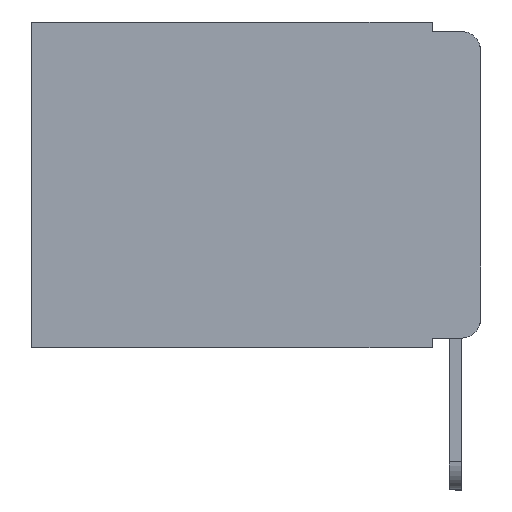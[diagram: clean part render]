
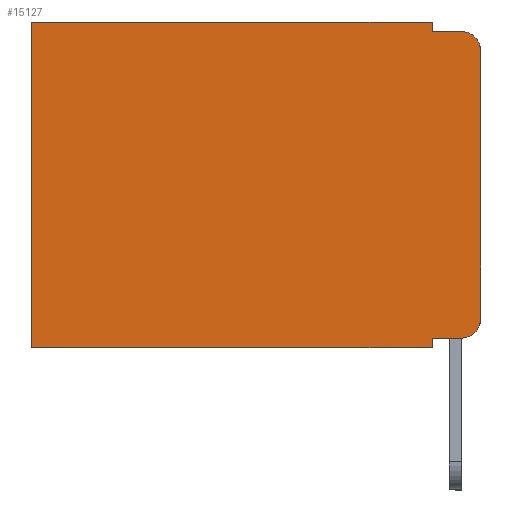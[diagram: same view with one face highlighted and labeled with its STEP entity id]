
A CAD part, left-side view. The second image highlights one B-rep face of the part: STEP entity #15127.
In plain terms, the highlighted planar face has unit normal (-1, 0, 0).
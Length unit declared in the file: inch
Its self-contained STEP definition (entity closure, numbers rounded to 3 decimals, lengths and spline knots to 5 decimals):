
#322 = CIRCLE ( 'NONE', #8937, 0.02 ) ;
#531 = VECTOR ( 'NONE', #4305, 39.37008 ) ;
#1271 = CARTESIAN_POINT ( 'NONE',  ( 0.298, 0.473, -0.343 ) ) ;
#1342 = CARTESIAN_POINT ( 'NONE',  ( 0.298, 0., -0.313 ) ) ;
#1642 = CARTESIAN_POINT ( 'NONE',  ( 0.298, 0.051, -0.01 ) ) ;
#1661 = CARTESIAN_POINT ( 'NONE',  ( 0.298, 0.473, 0. ) ) ;
#2006 = CARTESIAN_POINT ( 'NONE',  ( 0.298, 0., 0. ) ) ;
#2132 = LINE ( 'NONE', #8011, #18996 ) ;
#2340 = EDGE_CURVE ( 'NONE', #13632, #8010, #3094, .T. ) ;
#2547 = LINE ( 'NONE', #8413, #17342 ) ;
#2768 = ORIENTED_EDGE ( 'NONE', *, *, #10958, .T. ) ;
#2917 = LINE ( 'NONE', #5910, #15365 ) ;
#3084 = ORIENTED_EDGE ( 'NONE', *, *, #17409, .T. ) ;
#3089 = VERTEX_POINT ( 'NONE', #12776 ) ;
#3094 = LINE ( 'NONE', #4831, #15321 ) ;
#3151 = CARTESIAN_POINT ( 'NONE',  ( 0.298, 0.02, -0.03 ) ) ;
#3425 = CARTESIAN_POINT ( 'NONE',  ( 0.298, 0.473, 0. ) ) ;
#3670 = EDGE_CURVE ( 'NONE', #13991, #3089, #2132, .T. ) ;
#4305 = DIRECTION ( 'NONE',  ( 0., -1., 0. ) ) ;
#4351 = VERTEX_POINT ( 'NONE', #5762 ) ;
#4394 = EDGE_CURVE ( 'NONE', #13632, #5650, #15961, .T. ) ;
#4460 = DIRECTION ( 'NONE',  ( 0., 0., -1. ) ) ;
#4831 = CARTESIAN_POINT ( 'NONE',  ( 0.298, 0.051, 0. ) ) ;
#4907 = LINE ( 'NONE', #2006, #11786 ) ;
#5237 = ORIENTED_EDGE ( 'NONE', *, *, #5280, .F. ) ;
#5280 = EDGE_CURVE ( 'NONE', #8010, #14681, #2917, .T. ) ;
#5650 = VERTEX_POINT ( 'NONE', #11079 ) ;
#5762 = CARTESIAN_POINT ( 'NONE',  ( 0.298, 0.051, 0. ) ) ;
#5910 = CARTESIAN_POINT ( 'NONE',  ( 0.298, 0., -0.343 ) ) ;
#5914 = DIRECTION ( 'NONE',  ( -1., 0., 0. ) ) ;
#6096 = EDGE_CURVE ( 'NONE', #4351, #13991, #6538, .T. ) ;
#6273 = DIRECTION ( 'NONE',  ( 0., 0., -1. ) ) ;
#6279 = DIRECTION ( 'NONE',  ( 0., 0., -1. ) ) ;
#6538 = LINE ( 'NONE', #15402, #14755 ) ;
#7582 = DIRECTION ( 'NONE',  ( 0., 0., -1. ) ) ;
#7862 = DIRECTION ( 'NONE',  ( -1., 0., 0. ) ) ;
#8010 = VERTEX_POINT ( 'NONE', #13387 ) ;
#8011 = CARTESIAN_POINT ( 'NONE',  ( 0.298, 0.051, -0.01 ) ) ;
#8413 = CARTESIAN_POINT ( 'NONE',  ( 0.298, 0., 0. ) ) ;
#8636 = EDGE_CURVE ( 'NONE', #17493, #3089, #322, .T. ) ;
#8716 = VECTOR ( 'NONE', #11022, 39.37008 ) ;
#8937 = AXIS2_PLACEMENT_3D ( 'NONE', #3151, #7862, #7582 ) ;
#8964 = DIRECTION ( 'NONE',  ( 0., 1., 0. ) ) ;
#9158 = CARTESIAN_POINT ( 'NONE',  ( 0.298, 0.051, -0.333 ) ) ;
#9317 = EDGE_CURVE ( 'NONE', #5650, #13837, #17902, .T. ) ;
#10499 = DIRECTION ( 'NONE',  ( 1., 0., 0. ) ) ;
#10676 = DIRECTION ( 'NONE',  ( 0., 1., 0. ) ) ;
#10958 = EDGE_CURVE ( 'NONE', #4351, #12230, #4907, .T. ) ;
#11022 = DIRECTION ( 'NONE',  ( 0., 0., -1. ) ) ;
#11079 = CARTESIAN_POINT ( 'NONE',  ( 0.298, 0.02, -0.333 ) ) ;
#11455 = EDGE_CURVE ( 'NONE', #17493, #13837, #2547, .T. ) ;
#11786 = VECTOR ( 'NONE', #10676, 39.37008 ) ;
#11898 = ORIENTED_EDGE ( 'NONE', *, *, #3670, .F. ) ;
#11942 = ORIENTED_EDGE ( 'NONE', *, *, #2340, .F. ) ;
#12046 = CARTESIAN_POINT ( 'NONE',  ( 0.298, 0., 0. ) ) ;
#12054 = ORIENTED_EDGE ( 'NONE', *, *, #9317, .T. ) ;
#12230 = VERTEX_POINT ( 'NONE', #1661 ) ;
#12376 = LINE ( 'NONE', #3425, #8716 ) ;
#12776 = CARTESIAN_POINT ( 'NONE',  ( 0.298, 0.02, -0.01 ) ) ;
#13387 = CARTESIAN_POINT ( 'NONE',  ( 0.298, 0.051, -0.343 ) ) ;
#13491 = PLANE ( 'NONE',  #15713 ) ;
#13632 = VERTEX_POINT ( 'NONE', #9158 ) ;
#13704 = ORIENTED_EDGE ( 'NONE', *, *, #4394, .T. ) ;
#13822 = ORIENTED_EDGE ( 'NONE', *, *, #6096, .F. ) ;
#13837 = VERTEX_POINT ( 'NONE', #1342 ) ;
#13897 = DIRECTION ( 'NONE',  ( 0., -1., 0. ) ) ;
#13991 = VERTEX_POINT ( 'NONE', #1642 ) ;
#14556 = FACE_OUTER_BOUND ( 'NONE', #14898, .T. ) ;
#14681 = VERTEX_POINT ( 'NONE', #1271 ) ;
#14755 = VECTOR ( 'NONE', #18568, 39.37008 ) ;
#14860 = CARTESIAN_POINT ( 'NONE',  ( 0.298, 0.02, -0.313 ) ) ;
#14898 = EDGE_LOOP ( 'NONE', ( #15244, #18022, #11898, #13822, #2768, #3084, #5237, #11942, #13704, #12054 ) ) ;
#15127 = ADVANCED_FACE ( 'NONE', ( #14556 ), #13491, .F. ) ;
#15244 = ORIENTED_EDGE ( 'NONE', *, *, #11455, .F. ) ;
#15321 = VECTOR ( 'NONE', #6279, 39.37008 ) ;
#15365 = VECTOR ( 'NONE', #8964, 39.37008 ) ;
#15402 = CARTESIAN_POINT ( 'NONE',  ( 0.298, 0.051, 0. ) ) ;
#15681 = CARTESIAN_POINT ( 'NONE',  ( 0.298, 0.051, -0.333 ) ) ;
#15713 = AXIS2_PLACEMENT_3D ( 'NONE', #12046, #10499, #6273 ) ;
#15961 = LINE ( 'NONE', #15681, #531 ) ;
#17292 = DIRECTION ( 'NONE',  ( 0., 0., -1. ) ) ;
#17342 = VECTOR ( 'NONE', #17292, 39.37008 ) ;
#17409 = EDGE_CURVE ( 'NONE', #12230, #14681, #12376, .T. ) ;
#17493 = VERTEX_POINT ( 'NONE', #18064 ) ;
#17902 = CIRCLE ( 'NONE', #18497, 0.02 ) ;
#18022 = ORIENTED_EDGE ( 'NONE', *, *, #8636, .T. ) ;
#18064 = CARTESIAN_POINT ( 'NONE',  ( 0.298, 0., -0.03 ) ) ;
#18497 = AXIS2_PLACEMENT_3D ( 'NONE', #14860, #5914, #4460 ) ;
#18568 = DIRECTION ( 'NONE',  ( 0., 0., -1. ) ) ;
#18996 = VECTOR ( 'NONE', #13897, 39.37008 ) ;
